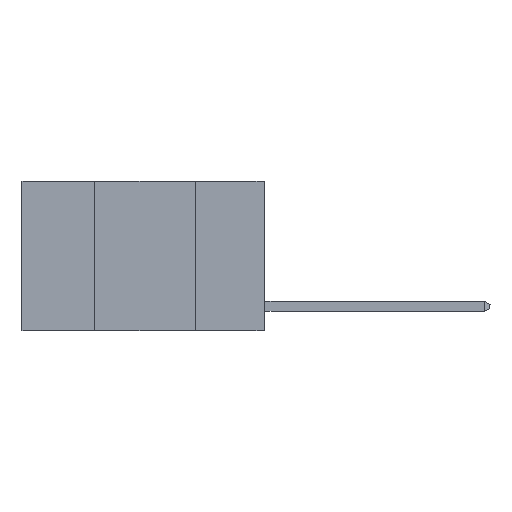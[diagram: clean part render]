
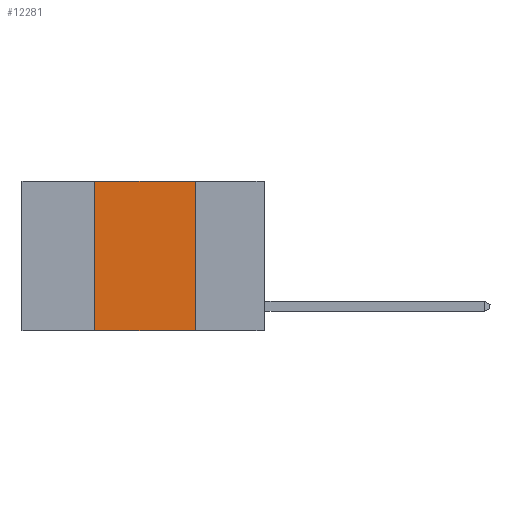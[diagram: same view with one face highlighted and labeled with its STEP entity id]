
A CAD part, left-side view. The second image highlights one B-rep face of the part: STEP entity #12281.
In plain terms, the highlighted planar face has unit normal (-1, 0, 0).
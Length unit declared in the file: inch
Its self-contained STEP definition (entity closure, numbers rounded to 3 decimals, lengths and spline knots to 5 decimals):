
#1222 = EDGE_CURVE ( 'NONE', #8628, #13828, #2260, .T. ) ;
#2260 = LINE ( 'NONE', #11288, #16693 ) ;
#2788 = CARTESIAN_POINT ( 'NONE',  ( 0., 0.6, 0. ) ) ;
#3271 = DIRECTION ( 'NONE',  ( 0., 0., -1. ) ) ;
#4845 = VERTEX_POINT ( 'NONE', #22548 ) ;
#4962 = DIRECTION ( 'NONE',  ( 0., -1., 0. ) ) ;
#6854 = EDGE_CURVE ( 'NONE', #4845, #16731, #22778, .T. ) ;
#8628 = VERTEX_POINT ( 'NONE', #14315 ) ;
#9545 = DIRECTION ( 'NONE',  ( 0., -1., 0. ) ) ;
#9769 = AXIS2_PLACEMENT_3D ( 'NONE', #2788, #16422, #18575 ) ;
#10535 = EDGE_CURVE ( 'NONE', #8628, #4845, #21969, .T. ) ;
#11288 = CARTESIAN_POINT ( 'NONE',  ( 0., 0.6, -0.37 ) ) ;
#12281 = ADVANCED_FACE ( 'NONE', ( #17935 ), #20544, .F. ) ;
#13828 = VERTEX_POINT ( 'NONE', #24793 ) ;
#14315 = CARTESIAN_POINT ( 'NONE',  ( 0., 0.42, -0.37 ) ) ;
#14649 = CARTESIAN_POINT ( 'NONE',  ( 0., 0.17, 0. ) ) ;
#15156 = ORIENTED_EDGE ( 'NONE', *, *, #24462, .F. ) ;
#16055 = VECTOR ( 'NONE', #3271, 39.37008 ) ;
#16422 = DIRECTION ( 'NONE',  ( 1., 0., 0. ) ) ;
#16693 = VECTOR ( 'NONE', #9545, 39.37008 ) ;
#16731 = VERTEX_POINT ( 'NONE', #14649 ) ;
#16767 = CARTESIAN_POINT ( 'NONE',  ( 0., 0.6, 0. ) ) ;
#16784 = EDGE_LOOP ( 'NONE', ( #15156, #19996, #17982, #18117 ) ) ;
#17935 = FACE_OUTER_BOUND ( 'NONE', #16784, .T. ) ;
#17982 = ORIENTED_EDGE ( 'NONE', *, *, #10535, .F. ) ;
#18117 = ORIENTED_EDGE ( 'NONE', *, *, #1222, .T. ) ;
#18575 = DIRECTION ( 'NONE',  ( 0., 0., -1. ) ) ;
#19679 = VECTOR ( 'NONE', #4962, 39.37008 ) ;
#19996 = ORIENTED_EDGE ( 'NONE', *, *, #6854, .F. ) ;
#20128 = VECTOR ( 'NONE', #23484, 39.37008 ) ;
#20329 = CARTESIAN_POINT ( 'NONE',  ( 0., 0.17, 0. ) ) ;
#20544 = PLANE ( 'NONE',  #9769 ) ;
#21969 = LINE ( 'NONE', #25274, #20128 ) ;
#22548 = CARTESIAN_POINT ( 'NONE',  ( 0., 0.42, 0. ) ) ;
#22778 = LINE ( 'NONE', #16767, #19679 ) ;
#23484 = DIRECTION ( 'NONE',  ( 0., 0., 1. ) ) ;
#24398 = LINE ( 'NONE', #20329, #16055 ) ;
#24462 = EDGE_CURVE ( 'NONE', #16731, #13828, #24398, .T. ) ;
#24793 = CARTESIAN_POINT ( 'NONE',  ( 0., 0.17, -0.37 ) ) ;
#25274 = CARTESIAN_POINT ( 'NONE',  ( 0., 0.42, 0. ) ) ;
